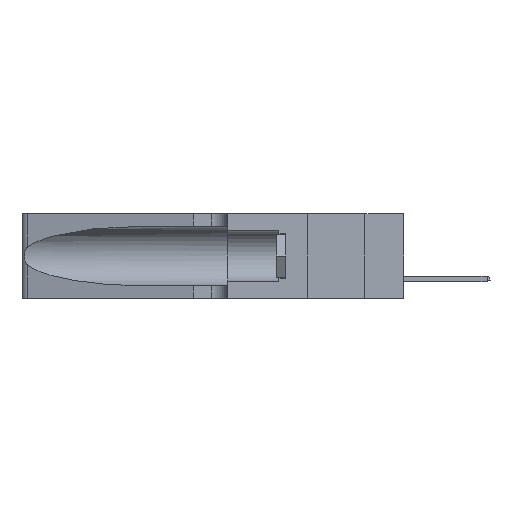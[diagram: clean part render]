
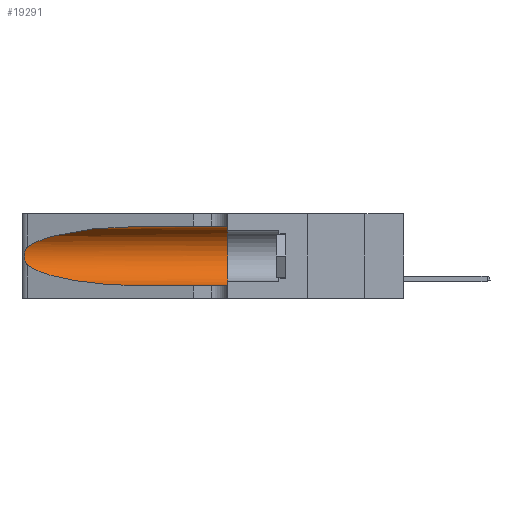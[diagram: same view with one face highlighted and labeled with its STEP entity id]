
A CAD part, left-side view. The second image highlights one B-rep face of the part: STEP entity #19291.
In plain terms, the highlighted cylindrical face has radius 3.308 mm (diameter 6.617 mm), a partial arc.
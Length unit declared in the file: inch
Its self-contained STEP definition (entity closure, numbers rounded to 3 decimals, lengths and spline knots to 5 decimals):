
#605 = CARTESIAN_POINT ( 'NONE',  ( 0.25639, 1.23186, 0.15144 ) ) ;
#1562 = ORIENTED_EDGE ( 'NONE', *, *, #23503, .F. ) ;
#1675 = EDGE_CURVE ( 'NONE', #22769, #16632, #21592, .T. ) ;
#2255 = CARTESIAN_POINT ( 'NONE',  ( 0.25487, 1.22718, 0.22369 ) ) ;
#2766 = CARTESIAN_POINT ( 'NONE',  ( 0.25487, 1.22718, 0.14631 ) ) ;
#3322 = CARTESIAN_POINT ( 'NONE',  ( 0.1305, 0.35, 0.31525 ) ) ;
#3789 = LINE ( 'NONE', #15822, #25908 ) ;
#3918 = CARTESIAN_POINT ( 'NONE',  ( 0.18966, 0.96281, 0.05475 ) ) ;
#4019 = CARTESIAN_POINT ( 'NONE',  ( 0.25487, 1.22718, 0.14631 ) ) ;
#4593 = B_SPLINE_CURVE_WITH_KNOTS ( 'NONE', 3,
 ( #26185, #20181, #9107, #11259, #17909, #15759, #26279, #17717, #9388, #11539, #13414, #605, #15575, #2766 ),
 .UNSPECIFIED., .F., .F.,
 ( 4, 2, 2, 2, 2, 2, 4 ),
 ( 0., 0.00027, 0.00053, 0.00107, 0.0016, 0.00187, 0.00214 ),
 .UNSPECIFIED. ) ;
#4652 = LINE ( 'NONE', #5605, #11316 ) ;
#4830 = EDGE_CURVE ( 'NONE', #22602, #24737, #4652, .T. ) ;
#5059 = DIRECTION ( 'NONE',  ( 0., -1., 0. ) ) ;
#5596 = ORIENTED_EDGE ( 'NONE', *, *, #1675, .T. ) ;
#5605 = CARTESIAN_POINT ( 'NONE',  ( 0.1305, 1.61858, 0.05475 ) ) ;
#5962 = CARTESIAN_POINT ( 'NONE',  ( 0.1305, 1.61858, 0.185 ) ) ;
#9107 = CARTESIAN_POINT ( 'NONE',  ( 0.25639, 1.23184, 0.21858 ) ) ;
#9388 = CARTESIAN_POINT ( 'NONE',  ( 0.26017, 1.23833, 0.17102 ) ) ;
#10007 = CYLINDRICAL_SURFACE ( 'NONE', #22984, 0.13025 ) ;
#10538 = CARTESIAN_POINT ( 'NONE',  ( 0.2373, 1.15595, 0.08982 ) ) ;
#10556 = CARTESIAN_POINT ( 'NONE',  ( 0.2373, 1.15595, 0.28018 ) ) ;
#10636 = CARTESIAN_POINT ( 'NONE',  ( 0.1305, 0.72297, 0.05475 ) ) ;
#11259 = CARTESIAN_POINT ( 'NONE',  ( 0.25787, 1.23484, 0.2124 ) ) ;
#11316 = VECTOR ( 'NONE', #22660, 39.37008 ) ;
#11407 = CARTESIAN_POINT ( 'NONE',  ( 0.25487, 1.22718, 0.14631 ) ) ;
#11539 = CARTESIAN_POINT ( 'NONE',  ( 0.25856, 1.23593, 0.16098 ) ) ;
#11648 = AXIS2_PLACEMENT_3D ( 'NONE', #13350, #19926, #17374 ) ;
#13350 = CARTESIAN_POINT ( 'NONE',  ( 0.1305, 0.35, 0.185 ) ) ;
#13414 = CARTESIAN_POINT ( 'NONE',  ( 0.25789, 1.23486, 0.15765 ) ) ;
#13641 = EDGE_CURVE ( 'NONE', #23533, #22602, #25715, .T. ) ;
#14466 = ORIENTED_EDGE ( 'NONE', *, *, #4830, .T. ) ;
#14825 = ORIENTED_EDGE ( 'NONE', *, *, #17981, .F. ) ;
#14937 = DIRECTION ( 'NONE',  ( 0., -1., 0. ) ) ;
#15375 = CARTESIAN_POINT ( 'NONE',  ( 0.1305, 0.72297, 0.31525 ) ) ;
#15575 = CARTESIAN_POINT ( 'NONE',  ( 0.25555, 1.22993, 0.14849 ) ) ;
#15759 = CARTESIAN_POINT ( 'NONE',  ( 0.26018, 1.23835, 0.19895 ) ) ;
#15822 = CARTESIAN_POINT ( 'NONE',  ( 0.1305, 1.61858, 0.31525 ) ) ;
#16632 = VERTEX_POINT ( 'NONE', #25364 ) ;
#17374 = DIRECTION ( 'NONE',  ( 0., 0., 1. ) ) ;
#17440 = CARTESIAN_POINT ( 'NONE',  ( 0.1305, 0.35, 0.05475 ) ) ;
#17548 = EDGE_LOOP ( 'NONE', ( #5596, #24703, #24211, #14466, #14825, #1562 ) ) ;
#17717 = CARTESIAN_POINT ( 'NONE',  ( 0.26075, 1.23896, 0.178 ) ) ;
#17909 = CARTESIAN_POINT ( 'NONE',  ( 0.25854, 1.2359, 0.20912 ) ) ;
#17981 = EDGE_CURVE ( 'NONE', #18101, #24737, #26910, .T. ) ;
#18101 = VERTEX_POINT ( 'NONE', #3322 ) ;
#19291 = ADVANCED_FACE ( 'NONE', ( #21092 ), #10007, .F. ) ;
#19926 = DIRECTION ( 'NONE',  ( 0., 1., 0. ) ) ;
#20181 = CARTESIAN_POINT ( 'NONE',  ( 0.25555, 1.22994, 0.2215 ) ) ;
#21092 = FACE_OUTER_BOUND ( 'NONE', #17548, .T. ) ;
#21330 = DIRECTION ( 'NONE',  ( 0., 0., -1. ) ) ;
#21592 =( BOUNDED_CURVE ( )  B_SPLINE_CURVE ( 3, ( #23507, #22014, #10556, #2255 ),
 .UNSPECIFIED., .F., .T. ) 
 B_SPLINE_CURVE_WITH_KNOTS ( ( 4, 4 ),
 ( 1.5708, 2.84003 ),
 .UNSPECIFIED. ) 
 CURVE ( )  GEOMETRIC_REPRESENTATION_ITEM ( )  RATIONAL_B_SPLINE_CURVE ( ( 1., 0.87, 0.87, 1. ) ) 
 REPRESENTATION_ITEM ( '' )  );
#22014 = CARTESIAN_POINT ( 'NONE',  ( 0.18966, 0.96281, 0.31525 ) ) ;
#22602 = VERTEX_POINT ( 'NONE', #23464 ) ;
#22660 = DIRECTION ( 'NONE',  ( 0., -1., 0. ) ) ;
#22769 = VERTEX_POINT ( 'NONE', #15375 ) ;
#22984 = AXIS2_PLACEMENT_3D ( 'NONE', #5962, #14937, #21330 ) ;
#23464 = CARTESIAN_POINT ( 'NONE',  ( 0.1305, 0.72297, 0.05475 ) ) ;
#23503 = EDGE_CURVE ( 'NONE', #22769, #18101, #3789, .T. ) ;
#23507 = CARTESIAN_POINT ( 'NONE',  ( 0.1305, 0.72297, 0.31525 ) ) ;
#23533 = VERTEX_POINT ( 'NONE', #11407 ) ;
#24211 = ORIENTED_EDGE ( 'NONE', *, *, #13641, .T. ) ;
#24703 = ORIENTED_EDGE ( 'NONE', *, *, #24905, .T. ) ;
#24737 = VERTEX_POINT ( 'NONE', #17440 ) ;
#24905 = EDGE_CURVE ( 'NONE', #16632, #23533, #4593, .T. ) ;
#25364 = CARTESIAN_POINT ( 'NONE',  ( 0.25487, 1.22718, 0.22369 ) ) ;
#25715 =( BOUNDED_CURVE ( )  B_SPLINE_CURVE ( 3, ( #4019, #10538, #3918, #10636 ),
 .UNSPECIFIED., .F., .F. ) 
 B_SPLINE_CURVE_WITH_KNOTS ( ( 4, 4 ),
 ( 3.44316, 4.71239 ),
 .UNSPECIFIED. ) 
 CURVE ( )  GEOMETRIC_REPRESENTATION_ITEM ( )  RATIONAL_B_SPLINE_CURVE ( ( 1., 0.87, 0.87, 1. ) ) 
 REPRESENTATION_ITEM ( '' )  );
#25908 = VECTOR ( 'NONE', #5059, 39.37008 ) ;
#26185 = CARTESIAN_POINT ( 'NONE',  ( 0.25487, 1.22718, 0.22369 ) ) ;
#26279 = CARTESIAN_POINT ( 'NONE',  ( 0.26075, 1.23896, 0.19203 ) ) ;
#26910 = CIRCLE ( 'NONE', #11648, 0.13025 ) ;
